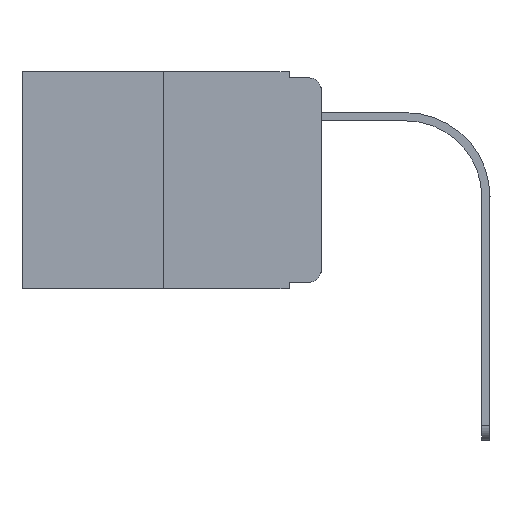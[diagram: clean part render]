
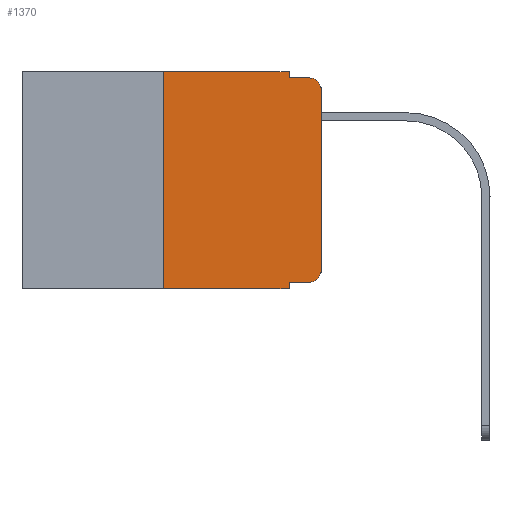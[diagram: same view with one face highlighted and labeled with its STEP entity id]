
A CAD part, left-side view. The second image highlights one B-rep face of the part: STEP entity #1370.
In plain terms, the highlighted planar face has unit normal (-1, 0, 0).
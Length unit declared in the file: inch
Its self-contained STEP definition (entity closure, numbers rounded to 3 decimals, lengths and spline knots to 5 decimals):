
#277 = EDGE_CURVE ( 'NONE', #11272, #14171, #22160, .T. ) ;
#906 = ORIENTED_EDGE ( 'NONE', *, *, #15935, .T. ) ;
#1358 = VERTEX_POINT ( 'NONE', #14526 ) ;
#1370 = ADVANCED_FACE ( 'NONE', ( #16261 ), #5683, .F. ) ;
#2445 = DIRECTION ( 'NONE',  ( 1., 0., 0. ) ) ;
#2515 = VECTOR ( 'NONE', #15881, 39.37008 ) ;
#2976 = CARTESIAN_POINT ( 'NONE',  ( 0., 0.051, -0.01 ) ) ;
#3655 = VECTOR ( 'NONE', #4986, 39.37008 ) ;
#3836 = VERTEX_POINT ( 'NONE', #5930 ) ;
#4137 = CARTESIAN_POINT ( 'NONE',  ( 0., 0.051, -0.333 ) ) ;
#4333 = LINE ( 'NONE', #11595, #20917 ) ;
#4513 = VECTOR ( 'NONE', #4929, 39.37008 ) ;
#4929 = DIRECTION ( 'NONE',  ( 0., -1., 0. ) ) ;
#4986 = DIRECTION ( 'NONE',  ( 0., -1., 0. ) ) ;
#5326 = LINE ( 'NONE', #15781, #3655 ) ;
#5683 = PLANE ( 'NONE',  #8632 ) ;
#5745 = CARTESIAN_POINT ( 'NONE',  ( 0., 0.051, -0.333 ) ) ;
#5805 = EDGE_CURVE ( 'NONE', #11907, #3836, #14865, .T. ) ;
#5920 = DIRECTION ( 'NONE',  ( 0., 0., -1. ) ) ;
#5923 = VECTOR ( 'NONE', #19942, 39.37008 ) ;
#5930 = CARTESIAN_POINT ( 'NONE',  ( 0., 0.051, -0.01 ) ) ;
#6380 = DIRECTION ( 'NONE',  ( 0., 0., -1. ) ) ;
#6453 = LINE ( 'NONE', #2976, #4513 ) ;
#6705 = LINE ( 'NONE', #19281, #17738 ) ;
#6810 = DIRECTION ( 'NONE',  ( 0., -1., 0. ) ) ;
#7066 = AXIS2_PLACEMENT_3D ( 'NONE', #7900, #9475, #9267 ) ;
#7216 = ORIENTED_EDGE ( 'NONE', *, *, #277, .T. ) ;
#7477 = VERTEX_POINT ( 'NONE', #5745 ) ;
#7900 = CARTESIAN_POINT ( 'NONE',  ( 0., 0.02, -0.03 ) ) ;
#7961 = EDGE_CURVE ( 'NONE', #1358, #20345, #17087, .T. ) ;
#8133 = ORIENTED_EDGE ( 'NONE', *, *, #5805, .F. ) ;
#8517 = ORIENTED_EDGE ( 'NONE', *, *, #17060, .T. ) ;
#8561 = EDGE_CURVE ( 'NONE', #3836, #11384, #6453, .T. ) ;
#8627 = VERTEX_POINT ( 'NONE', #20842 ) ;
#8632 = AXIS2_PLACEMENT_3D ( 'NONE', #14626, #2445, #5920 ) ;
#9171 = ORIENTED_EDGE ( 'NONE', *, *, #20174, .F. ) ;
#9267 = DIRECTION ( 'NONE',  ( 0., 0., -1. ) ) ;
#9475 = DIRECTION ( 'NONE',  ( -1., 0., 0. ) ) ;
#9598 = ORIENTED_EDGE ( 'NONE', *, *, #8561, .F. ) ;
#9807 = DIRECTION ( 'NONE',  ( 0., 0., 1. ) ) ;
#9973 = CARTESIAN_POINT ( 'NONE',  ( 0., 0.25, 0. ) ) ;
#10496 = CARTESIAN_POINT ( 'NONE',  ( 0., 0., -0.313 ) ) ;
#10600 = CARTESIAN_POINT ( 'NONE',  ( 0., 0.051, -0.343 ) ) ;
#10758 = CARTESIAN_POINT ( 'NONE',  ( 0., 0., -0.03 ) ) ;
#11272 = VERTEX_POINT ( 'NONE', #10496 ) ;
#11384 = VERTEX_POINT ( 'NONE', #17825 ) ;
#11595 = CARTESIAN_POINT ( 'NONE',  ( 0., 0.051, 0. ) ) ;
#11841 = AXIS2_PLACEMENT_3D ( 'NONE', #12234, #17934, #19412 ) ;
#11888 = CARTESIAN_POINT ( 'NONE',  ( 0., 0., 0. ) ) ;
#11907 = VERTEX_POINT ( 'NONE', #20594 ) ;
#11962 = EDGE_CURVE ( 'NONE', #20345, #11907, #5326, .T. ) ;
#11996 = ORIENTED_EDGE ( 'NONE', *, *, #13328, .T. ) ;
#12234 = CARTESIAN_POINT ( 'NONE',  ( 0., 0.02, -0.313 ) ) ;
#12567 = ORIENTED_EDGE ( 'NONE', *, *, #11962, .F. ) ;
#12864 = ORIENTED_EDGE ( 'NONE', *, *, #7961, .F. ) ;
#13328 = EDGE_CURVE ( 'NONE', #1358, #18237, #6705, .T. ) ;
#13457 = ORIENTED_EDGE ( 'NONE', *, *, #22431, .T. ) ;
#14011 = CARTESIAN_POINT ( 'NONE',  ( 0., 0.25, 0. ) ) ;
#14027 = EDGE_LOOP ( 'NONE', ( #7216, #13457, #9598, #8133, #12567, #12864, #11996, #9171, #8517, #906 ) ) ;
#14042 = CIRCLE ( 'NONE', #7066, 0.02 ) ;
#14147 = VECTOR ( 'NONE', #9807, 39.37008 ) ;
#14171 = VERTEX_POINT ( 'NONE', #10758 ) ;
#14526 = CARTESIAN_POINT ( 'NONE',  ( 0., 0.25, -0.343 ) ) ;
#14626 = CARTESIAN_POINT ( 'NONE',  ( 0., 0.473, 0. ) ) ;
#14865 = LINE ( 'NONE', #16935, #17600 ) ;
#15162 = DIRECTION ( 'NONE',  ( 0., 0., -1. ) ) ;
#15781 = CARTESIAN_POINT ( 'NONE',  ( 0., 0.473, 0. ) ) ;
#15881 = DIRECTION ( 'NONE',  ( 0., -1., 0. ) ) ;
#15935 = EDGE_CURVE ( 'NONE', #8627, #11272, #16230, .T. ) ;
#16230 = CIRCLE ( 'NONE', #11841, 0.02 ) ;
#16261 = FACE_OUTER_BOUND ( 'NONE', #14027, .T. ) ;
#16935 = CARTESIAN_POINT ( 'NONE',  ( 0., 0.051, 0. ) ) ;
#17060 = EDGE_CURVE ( 'NONE', #7477, #8627, #21545, .T. ) ;
#17087 = LINE ( 'NONE', #9973, #5923 ) ;
#17600 = VECTOR ( 'NONE', #6380, 39.37008 ) ;
#17738 = VECTOR ( 'NONE', #6810, 39.37008 ) ;
#17825 = CARTESIAN_POINT ( 'NONE',  ( 0., 0.02, -0.01 ) ) ;
#17934 = DIRECTION ( 'NONE',  ( -1., 0., 0. ) ) ;
#18237 = VERTEX_POINT ( 'NONE', #10600 ) ;
#19281 = CARTESIAN_POINT ( 'NONE',  ( 0., 0.473, -0.343 ) ) ;
#19412 = DIRECTION ( 'NONE',  ( 0., 0., -1. ) ) ;
#19942 = DIRECTION ( 'NONE',  ( 0., 0., 1. ) ) ;
#20174 = EDGE_CURVE ( 'NONE', #7477, #18237, #4333, .T. ) ;
#20345 = VERTEX_POINT ( 'NONE', #14011 ) ;
#20594 = CARTESIAN_POINT ( 'NONE',  ( 0., 0.051, 0. ) ) ;
#20842 = CARTESIAN_POINT ( 'NONE',  ( 0., 0.02, -0.333 ) ) ;
#20917 = VECTOR ( 'NONE', #15162, 39.37008 ) ;
#21545 = LINE ( 'NONE', #4137, #2515 ) ;
#22160 = LINE ( 'NONE', #11888, #14147 ) ;
#22431 = EDGE_CURVE ( 'NONE', #14171, #11384, #14042, .T. ) ;
